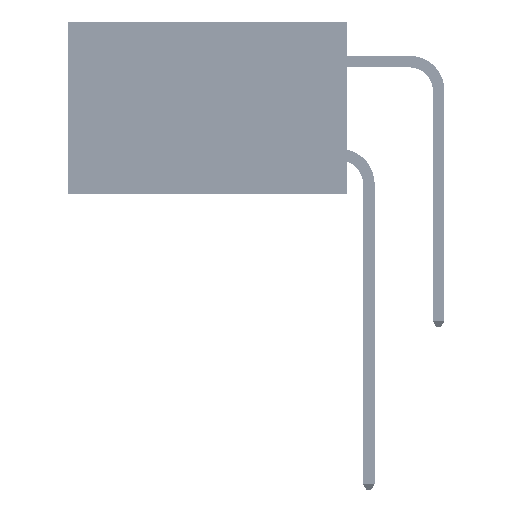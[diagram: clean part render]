
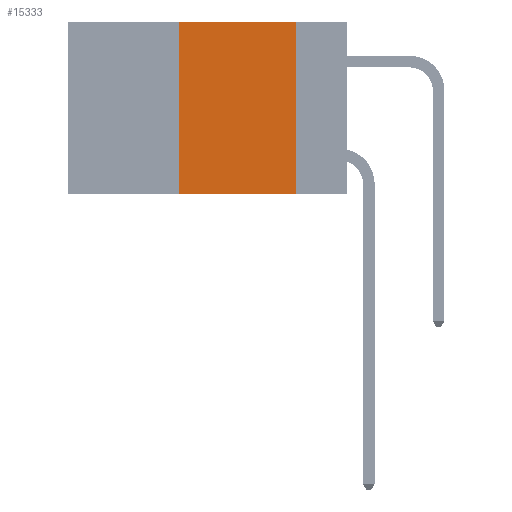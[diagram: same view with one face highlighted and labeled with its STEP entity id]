
A CAD part, left-side view. The second image highlights one B-rep face of the part: STEP entity #15333.
In plain terms, the highlighted planar face has unit normal (-1, 0, 0).
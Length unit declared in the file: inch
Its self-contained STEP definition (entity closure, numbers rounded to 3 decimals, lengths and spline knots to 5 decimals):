
#76 = CARTESIAN_POINT ( 'NONE',  ( 0., 0.6, 0. ) ) ;
#1243 = DIRECTION ( 'NONE',  ( 0., -1., 0. ) ) ;
#2086 = CARTESIAN_POINT ( 'NONE',  ( 0., 0.11, -0.37 ) ) ;
#4316 = ORIENTED_EDGE ( 'NONE', *, *, #30471, .F. ) ;
#7921 = VECTOR ( 'NONE', #21737, 39.37008 ) ;
#8594 = ORIENTED_EDGE ( 'NONE', *, *, #25944, .F. ) ;
#15074 = CARTESIAN_POINT ( 'NONE',  ( 0., 0.36, -0.37 ) ) ;
#15261 = AXIS2_PLACEMENT_3D ( 'NONE', #19991, #24053, #45131 ) ;
#15333 = ADVANCED_FACE ( 'NONE', ( #48368 ), #44589, .F. ) ;
#16752 = CARTESIAN_POINT ( 'NONE',  ( 0., 0.36, 0. ) ) ;
#17437 = ORIENTED_EDGE ( 'NONE', *, *, #20584, .F. ) ;
#19991 = CARTESIAN_POINT ( 'NONE',  ( 0., 0.6, 0. ) ) ;
#20361 = LINE ( 'NONE', #76, #27181 ) ;
#20584 = EDGE_CURVE ( 'NONE', #25581, #42548, #45914, .T. ) ;
#20720 = VERTEX_POINT ( 'NONE', #2086 ) ;
#21708 = EDGE_LOOP ( 'NONE', ( #8594, #4316, #17437, #34666 ) ) ;
#21737 = DIRECTION ( 'NONE',  ( 0., 0., -1. ) ) ;
#23874 = DIRECTION ( 'NONE',  ( 0., -1., 0. ) ) ;
#24053 = DIRECTION ( 'NONE',  ( 1., 0., 0. ) ) ;
#25581 = VERTEX_POINT ( 'NONE', #15074 ) ;
#25944 = EDGE_CURVE ( 'NONE', #31548, #20720, #46340, .T. ) ;
#27181 = VECTOR ( 'NONE', #23874, 39.37008 ) ;
#28616 = CARTESIAN_POINT ( 'NONE',  ( 0., 0.36, 0. ) ) ;
#30471 = EDGE_CURVE ( 'NONE', #42548, #31548, #20361, .T. ) ;
#31548 = VERTEX_POINT ( 'NONE', #33420 ) ;
#33420 = CARTESIAN_POINT ( 'NONE',  ( 0., 0.11, 0. ) ) ;
#34666 = ORIENTED_EDGE ( 'NONE', *, *, #51867, .T. ) ;
#42057 = LINE ( 'NONE', #42851, #50132 ) ;
#42100 = VECTOR ( 'NONE', #45652, 39.37008 ) ;
#42548 = VERTEX_POINT ( 'NONE', #28616 ) ;
#42851 = CARTESIAN_POINT ( 'NONE',  ( 0., 0.6, -0.37 ) ) ;
#44589 = PLANE ( 'NONE',  #15261 ) ;
#45131 = DIRECTION ( 'NONE',  ( 0., 0., -1. ) ) ;
#45652 = DIRECTION ( 'NONE',  ( 0., 0., 1. ) ) ;
#45914 = LINE ( 'NONE', #16752, #42100 ) ;
#46340 = LINE ( 'NONE', #46605, #7921 ) ;
#46605 = CARTESIAN_POINT ( 'NONE',  ( 0., 0.11, 0. ) ) ;
#48368 = FACE_OUTER_BOUND ( 'NONE', #21708, .T. ) ;
#50132 = VECTOR ( 'NONE', #1243, 39.37008 ) ;
#51867 = EDGE_CURVE ( 'NONE', #25581, #20720, #42057, .T. ) ;
